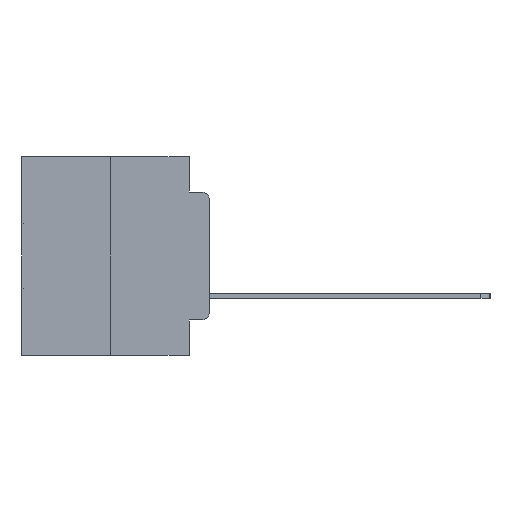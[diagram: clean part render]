
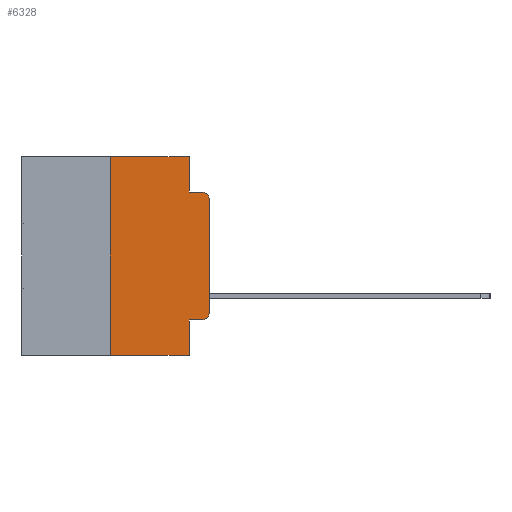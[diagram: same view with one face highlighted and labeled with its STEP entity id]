
A CAD part, left-side view. The second image highlights one B-rep face of the part: STEP entity #6328.
In plain terms, the highlighted planar face has unit normal (-1, 0, 0).
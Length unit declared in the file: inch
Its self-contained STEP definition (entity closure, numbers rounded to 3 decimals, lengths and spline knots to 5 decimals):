
#964 = VECTOR ( 'NONE', #25776, 39.37008 ) ;
#1037 = DIRECTION ( 'NONE',  ( 0., 0., 1. ) ) ;
#1412 = CARTESIAN_POINT ( 'NONE',  ( 0., 0.25, 0. ) ) ;
#2305 = VECTOR ( 'NONE', #18268, 39.37008 ) ;
#2512 = VERTEX_POINT ( 'NONE', #15554 ) ;
#2690 = CARTESIAN_POINT ( 'NONE',  ( 0., 0.051, -0.5 ) ) ;
#3006 = PLANE ( 'NONE',  #19744 ) ;
#3024 = LINE ( 'NONE', #9250, #2305 ) ;
#3517 = VERTEX_POINT ( 'NONE', #25816 ) ;
#4092 = VECTOR ( 'NONE', #25306, 39.37008 ) ;
#4685 = EDGE_CURVE ( 'NONE', #26063, #15414, #20037, .T. ) ;
#5258 = ORIENTED_EDGE ( 'NONE', *, *, #26778, .F. ) ;
#5262 = EDGE_CURVE ( 'NONE', #2512, #26063, #16503, .T. ) ;
#5438 = ORIENTED_EDGE ( 'NONE', *, *, #21425, .T. ) ;
#5967 = DIRECTION ( 'NONE',  ( -1., 0., 0. ) ) ;
#6193 = CARTESIAN_POINT ( 'NONE',  ( 0., 0.473, 0. ) ) ;
#6328 = ADVANCED_FACE ( 'NONE', ( #28643 ), #3006, .F. ) ;
#6981 = EDGE_CURVE ( 'NONE', #15324, #17799, #23744, .T. ) ;
#7017 = LINE ( 'NONE', #14568, #964 ) ;
#7449 = EDGE_LOOP ( 'NONE', ( #5438, #21314, #17760, #5258, #16499, #21872, #19716, #18811, #11203, #24513 ) ) ;
#7564 = DIRECTION ( 'NONE',  ( 1., 0., 0. ) ) ;
#8096 = VECTOR ( 'NONE', #28588, 39.37008 ) ;
#8315 = CARTESIAN_POINT ( 'NONE',  ( 0., 0.25, 0. ) ) ;
#9157 = EDGE_CURVE ( 'NONE', #9424, #17799, #16069, .T. ) ;
#9250 = CARTESIAN_POINT ( 'NONE',  ( 0., 0.051, 0. ) ) ;
#9424 = VERTEX_POINT ( 'NONE', #17418 ) ;
#10592 = DIRECTION ( 'NONE',  ( 0., 0., 1. ) ) ;
#11134 = AXIS2_PLACEMENT_3D ( 'NONE', #26300, #12914, #28533 ) ;
#11203 = ORIENTED_EDGE ( 'NONE', *, *, #18861, .T. ) ;
#12207 = LINE ( 'NONE', #14585, #18169 ) ;
#12839 = CARTESIAN_POINT ( 'NONE',  ( 0., 0.051, -0.4115 ) ) ;
#12882 = VERTEX_POINT ( 'NONE', #16084 ) ;
#12914 = DIRECTION ( 'NONE',  ( -1., 0., 0. ) ) ;
#13163 = CARTESIAN_POINT ( 'NONE',  ( 0., 0.051, 0. ) ) ;
#14359 = LINE ( 'NONE', #13163, #27625 ) ;
#14568 = CARTESIAN_POINT ( 'NONE',  ( 0., 0.473, -0.5 ) ) ;
#14585 = CARTESIAN_POINT ( 'NONE',  ( 0., 0., 0. ) ) ;
#14952 = EDGE_CURVE ( 'NONE', #3517, #17640, #16904, .T. ) ;
#15324 = VERTEX_POINT ( 'NONE', #27994 ) ;
#15414 = VERTEX_POINT ( 'NONE', #28371 ) ;
#15554 = CARTESIAN_POINT ( 'NONE',  ( 0., 0.25, -0.5 ) ) ;
#16069 = LINE ( 'NONE', #27547, #4092 ) ;
#16084 = CARTESIAN_POINT ( 'NONE',  ( 0., 0.051, -0.4115 ) ) ;
#16499 = ORIENTED_EDGE ( 'NONE', *, *, #4685, .F. ) ;
#16503 = LINE ( 'NONE', #8315, #26958 ) ;
#16904 = CIRCLE ( 'NONE', #17004, 0.02 ) ;
#16971 = EDGE_CURVE ( 'NONE', #12882, #18555, #3024, .T. ) ;
#17004 = AXIS2_PLACEMENT_3D ( 'NONE', #19401, #5967, #21648 ) ;
#17366 = DIRECTION ( 'NONE',  ( 0., -1., 0. ) ) ;
#17418 = CARTESIAN_POINT ( 'NONE',  ( 0., 0.051, -0.0885 ) ) ;
#17640 = VERTEX_POINT ( 'NONE', #27681 ) ;
#17760 = ORIENTED_EDGE ( 'NONE', *, *, #9157, .F. ) ;
#17799 = VERTEX_POINT ( 'NONE', #28245 ) ;
#18169 = VECTOR ( 'NONE', #1037, 39.37008 ) ;
#18268 = DIRECTION ( 'NONE',  ( 0., 0., -1. ) ) ;
#18555 = VERTEX_POINT ( 'NONE', #2690 ) ;
#18811 = ORIENTED_EDGE ( 'NONE', *, *, #16971, .F. ) ;
#18861 = EDGE_CURVE ( 'NONE', #12882, #3517, #21606, .T. ) ;
#19401 = CARTESIAN_POINT ( 'NONE',  ( 0., 0.02, -0.3915 ) ) ;
#19716 = ORIENTED_EDGE ( 'NONE', *, *, #25969, .T. ) ;
#19744 = AXIS2_PLACEMENT_3D ( 'NONE', #27624, #7564, #23253 ) ;
#20037 = LINE ( 'NONE', #6193, #8096 ) ;
#21314 = ORIENTED_EDGE ( 'NONE', *, *, #6981, .T. ) ;
#21425 = EDGE_CURVE ( 'NONE', #17640, #15324, #12207, .T. ) ;
#21606 = LINE ( 'NONE', #12839, #27518 ) ;
#21648 = DIRECTION ( 'NONE',  ( 0., 0., -1. ) ) ;
#21872 = ORIENTED_EDGE ( 'NONE', *, *, #5262, .F. ) ;
#23253 = DIRECTION ( 'NONE',  ( 0., 0., -1. ) ) ;
#23744 = CIRCLE ( 'NONE', #11134, 0.02 ) ;
#24513 = ORIENTED_EDGE ( 'NONE', *, *, #14952, .T. ) ;
#25306 = DIRECTION ( 'NONE',  ( 0., -1., 0. ) ) ;
#25776 = DIRECTION ( 'NONE',  ( 0., -1., 0. ) ) ;
#25816 = CARTESIAN_POINT ( 'NONE',  ( 0., 0.02, -0.4115 ) ) ;
#25969 = EDGE_CURVE ( 'NONE', #2512, #18555, #7017, .T. ) ;
#26063 = VERTEX_POINT ( 'NONE', #1412 ) ;
#26300 = CARTESIAN_POINT ( 'NONE',  ( 0., 0.02, -0.1085 ) ) ;
#26536 = DIRECTION ( 'NONE',  ( 0., 0., -1. ) ) ;
#26778 = EDGE_CURVE ( 'NONE', #15414, #9424, #14359, .T. ) ;
#26958 = VECTOR ( 'NONE', #10592, 39.37008 ) ;
#27518 = VECTOR ( 'NONE', #17366, 39.37008 ) ;
#27547 = CARTESIAN_POINT ( 'NONE',  ( 0., 0.051, -0.0885 ) ) ;
#27624 = CARTESIAN_POINT ( 'NONE',  ( 0., 0.473, 0. ) ) ;
#27625 = VECTOR ( 'NONE', #26536, 39.37008 ) ;
#27681 = CARTESIAN_POINT ( 'NONE',  ( 0., 0., -0.3915 ) ) ;
#27994 = CARTESIAN_POINT ( 'NONE',  ( 0., 0., -0.1085 ) ) ;
#28245 = CARTESIAN_POINT ( 'NONE',  ( 0., 0.02, -0.0885 ) ) ;
#28371 = CARTESIAN_POINT ( 'NONE',  ( 0., 0.051, 0. ) ) ;
#28533 = DIRECTION ( 'NONE',  ( 0., 0., -1. ) ) ;
#28588 = DIRECTION ( 'NONE',  ( 0., -1., 0. ) ) ;
#28643 = FACE_OUTER_BOUND ( 'NONE', #7449, .T. ) ;
